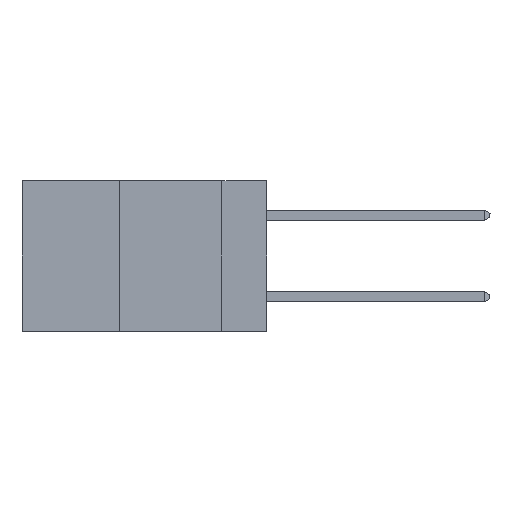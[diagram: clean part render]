
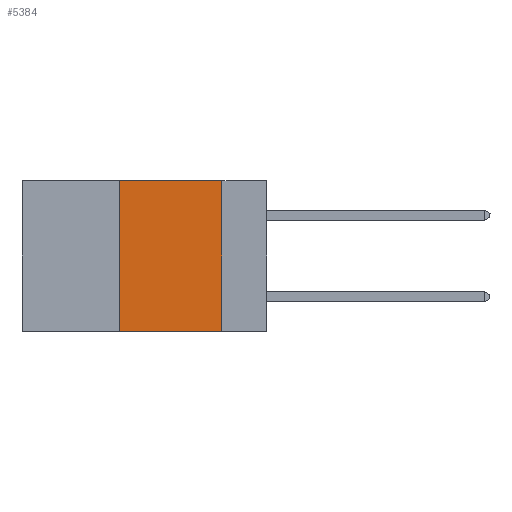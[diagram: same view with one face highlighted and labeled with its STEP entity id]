
A CAD part, left-side view. The second image highlights one B-rep face of the part: STEP entity #5384.
In plain terms, the highlighted planar face has unit normal (-1, 0, 0).
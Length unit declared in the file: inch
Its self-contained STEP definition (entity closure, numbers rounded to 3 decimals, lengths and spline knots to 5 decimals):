
#33 = EDGE_LOOP ( 'NONE', ( #14499, #4248, #11411, #13243 ) ) ;
#53 = DIRECTION ( 'NONE',  ( 0., -1., 0. ) ) ;
#418 = LINE ( 'NONE', #14309, #4543 ) ;
#489 = EDGE_CURVE ( 'NONE', #2208, #8171, #418, .T. ) ;
#653 = CARTESIAN_POINT ( 'NONE',  ( 0., 0.36, 0. ) ) ;
#1597 = DIRECTION ( 'NONE',  ( 0., 0., -1. ) ) ;
#1793 = CARTESIAN_POINT ( 'NONE',  ( 0., 0.6, 0. ) ) ;
#2115 = DIRECTION ( 'NONE',  ( 0., -1., 0. ) ) ;
#2208 = VERTEX_POINT ( 'NONE', #6661 ) ;
#4248 = ORIENTED_EDGE ( 'NONE', *, *, #19505, .F. ) ;
#4443 = LINE ( 'NONE', #18056, #4969 ) ;
#4543 = VECTOR ( 'NONE', #2115, 39.37008 ) ;
#4969 = VECTOR ( 'NONE', #7375, 39.37008 ) ;
#5384 = ADVANCED_FACE ( 'NONE', ( #10871 ), #13797, .F. ) ;
#6316 = DIRECTION ( 'NONE',  ( 1., 0., 0. ) ) ;
#6649 = AXIS2_PLACEMENT_3D ( 'NONE', #1793, #6316, #1597 ) ;
#6661 = CARTESIAN_POINT ( 'NONE',  ( 0., 0.36, -0.37 ) ) ;
#7103 = CARTESIAN_POINT ( 'NONE',  ( 0., 0.36, 0. ) ) ;
#7375 = DIRECTION ( 'NONE',  ( 0., 0., -1. ) ) ;
#8171 = VERTEX_POINT ( 'NONE', #19215 ) ;
#8793 = VERTEX_POINT ( 'NONE', #7103 ) ;
#10871 = FACE_OUTER_BOUND ( 'NONE', #33, .T. ) ;
#11093 = EDGE_CURVE ( 'NONE', #19592, #8171, #4443, .T. ) ;
#11148 = LINE ( 'NONE', #653, #16311 ) ;
#11250 = VECTOR ( 'NONE', #53, 39.37008 ) ;
#11342 = DIRECTION ( 'NONE',  ( 0., 0., 1. ) ) ;
#11411 = ORIENTED_EDGE ( 'NONE', *, *, #15542, .F. ) ;
#12253 = CARTESIAN_POINT ( 'NONE',  ( 0., 0.6, 0. ) ) ;
#13243 = ORIENTED_EDGE ( 'NONE', *, *, #489, .T. ) ;
#13797 = PLANE ( 'NONE',  #6649 ) ;
#13947 = LINE ( 'NONE', #12253, #11250 ) ;
#14309 = CARTESIAN_POINT ( 'NONE',  ( 0., 0.6, -0.37 ) ) ;
#14499 = ORIENTED_EDGE ( 'NONE', *, *, #11093, .F. ) ;
#15542 = EDGE_CURVE ( 'NONE', #2208, #8793, #11148, .T. ) ;
#15951 = CARTESIAN_POINT ( 'NONE',  ( 0., 0.11, 0. ) ) ;
#16311 = VECTOR ( 'NONE', #11342, 39.37008 ) ;
#18056 = CARTESIAN_POINT ( 'NONE',  ( 0., 0.11, 0. ) ) ;
#19215 = CARTESIAN_POINT ( 'NONE',  ( 0., 0.11, -0.37 ) ) ;
#19505 = EDGE_CURVE ( 'NONE', #8793, #19592, #13947, .T. ) ;
#19592 = VERTEX_POINT ( 'NONE', #15951 ) ;
